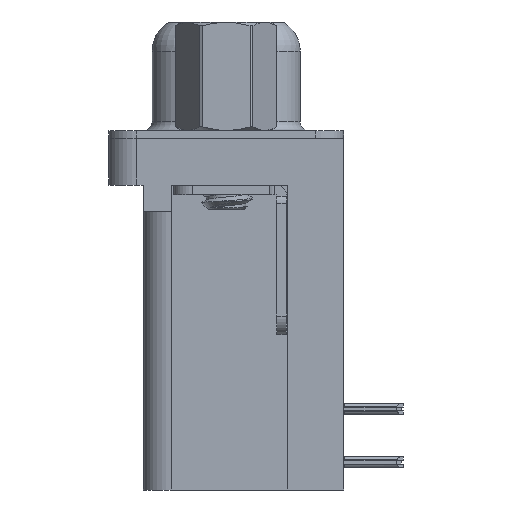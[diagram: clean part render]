
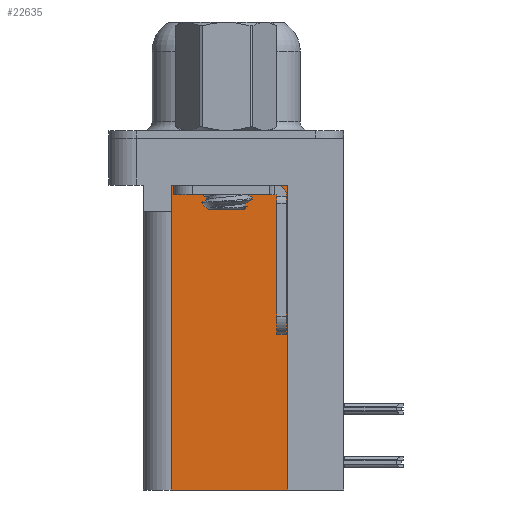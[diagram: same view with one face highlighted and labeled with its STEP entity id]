
A CAD part, left-side view. The second image highlights one B-rep face of the part: STEP entity #22635.
In plain terms, the highlighted planar face has unit normal (-1, 0, 0).
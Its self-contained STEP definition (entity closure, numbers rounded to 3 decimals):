
#1714 = CARTESIAN_POINT ( 'NONE',  ( 3.7, 2.925, -3.9 ) ) ;
#1843 = VERTEX_POINT ( 'NONE', #20753 ) ;
#1855 = ORIENTED_EDGE ( 'NONE', *, *, #30681, .T. ) ;
#2892 = VERTEX_POINT ( 'NONE', #13455 ) ;
#4314 = EDGE_LOOP ( 'NONE', ( #1855, #23134, #9907, #20919, #9679, #12378 ) ) ;
#4575 = DIRECTION ( 'NONE',  ( 0., 0., -1. ) ) ;
#5779 = VECTOR ( 'NONE', #31822, 1000. ) ;
#7782 = LINE ( 'NONE', #9061, #5779 ) ;
#8745 = PLANE ( 'NONE',  #29263 ) ;
#9061 = CARTESIAN_POINT ( 'NONE',  ( 3.7, 2.925, -18.76 ) ) ;
#9149 = VERTEX_POINT ( 'NONE', #28769 ) ;
#9576 = LINE ( 'NONE', #19725, #9988 ) ;
#9679 = ORIENTED_EDGE ( 'NONE', *, *, #22651, .F. ) ;
#9907 = ORIENTED_EDGE ( 'NONE', *, *, #19859, .T. ) ;
#9988 = VECTOR ( 'NONE', #4575, 1000. ) ;
#11217 = EDGE_CURVE ( 'NONE', #2892, #22349, #9576, .T. ) ;
#11319 = DIRECTION ( 'NONE',  ( 1., 0., 0. ) ) ;
#12378 = ORIENTED_EDGE ( 'NONE', *, *, #28851, .T. ) ;
#13455 = CARTESIAN_POINT ( 'NONE',  ( 3.7, 2.895, -2.5 ) ) ;
#14053 = CARTESIAN_POINT ( 'NONE',  ( 3.7, -3.295, -18.76 ) ) ;
#14070 = VERTEX_POINT ( 'NONE', #1714 ) ;
#14778 = CARTESIAN_POINT ( 'NONE',  ( 3.7, 0., -3.9 ) ) ;
#14834 = CARTESIAN_POINT ( 'NONE',  ( 3.7, -3.295, -18.76 ) ) ;
#15709 = VECTOR ( 'NONE', #22301, 1000. ) ;
#16117 = CARTESIAN_POINT ( 'NONE',  ( 3.7, -3.295, -2.5 ) ) ;
#16554 = DIRECTION ( 'NONE',  ( 0., 1., 0. ) ) ;
#17292 = LINE ( 'NONE', #14778, #15709 ) ;
#17494 = VERTEX_POINT ( 'NONE', #20575 ) ;
#18769 = CARTESIAN_POINT ( 'NONE',  ( 3.7, -3.295, -18.76 ) ) ;
#19610 = VECTOR ( 'NONE', #16554, 1000. ) ;
#19725 = CARTESIAN_POINT ( 'NONE',  ( 3.7, 2.895, -3.9 ) ) ;
#19859 = EDGE_CURVE ( 'NONE', #22349, #14070, #17292, .T. ) ;
#20027 = LINE ( 'NONE', #14053, #19610 ) ;
#20575 = CARTESIAN_POINT ( 'NONE',  ( 3.7, -3.295, -2.5 ) ) ;
#20753 = CARTESIAN_POINT ( 'NONE',  ( 3.7, 2.925, -18.76 ) ) ;
#20919 = ORIENTED_EDGE ( 'NONE', *, *, #21594, .F. ) ;
#21221 = FACE_OUTER_BOUND ( 'NONE', #4314, .T. ) ;
#21594 = EDGE_CURVE ( 'NONE', #1843, #14070, #7782, .T. ) ;
#22286 = VECTOR ( 'NONE', #24347, 1000. ) ;
#22301 = DIRECTION ( 'NONE',  ( 0., 1., 0. ) ) ;
#22349 = VERTEX_POINT ( 'NONE', #27643 ) ;
#22357 = LINE ( 'NONE', #16117, #22286 ) ;
#22635 = ADVANCED_FACE ( 'NONE', ( #21221 ), #8745, .F. ) ;
#22651 = EDGE_CURVE ( 'NONE', #9149, #1843, #20027, .T. ) ;
#23134 = ORIENTED_EDGE ( 'NONE', *, *, #11217, .T. ) ;
#24347 = DIRECTION ( 'NONE',  ( 0., 1., 0. ) ) ;
#24982 = DIRECTION ( 'NONE',  ( 0., 0., 1. ) ) ;
#27643 = CARTESIAN_POINT ( 'NONE',  ( 3.7, 2.895, -3.9 ) ) ;
#28769 = CARTESIAN_POINT ( 'NONE',  ( 3.7, -3.295, -18.76 ) ) ;
#28851 = EDGE_CURVE ( 'NONE', #9149, #17494, #29505, .T. ) ;
#29061 = DIRECTION ( 'NONE',  ( 0., 1., 0. ) ) ;
#29263 = AXIS2_PLACEMENT_3D ( 'NONE', #18769, #11319, #29061 ) ;
#29294 = VECTOR ( 'NONE', #24982, 1000. ) ;
#29505 = LINE ( 'NONE', #14834, #29294 ) ;
#30681 = EDGE_CURVE ( 'NONE', #17494, #2892, #22357, .T. ) ;
#31822 = DIRECTION ( 'NONE',  ( 0., 0., 1. ) ) ;
